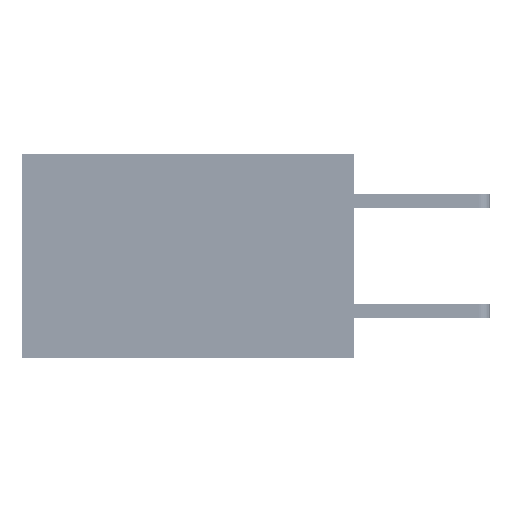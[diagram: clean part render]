
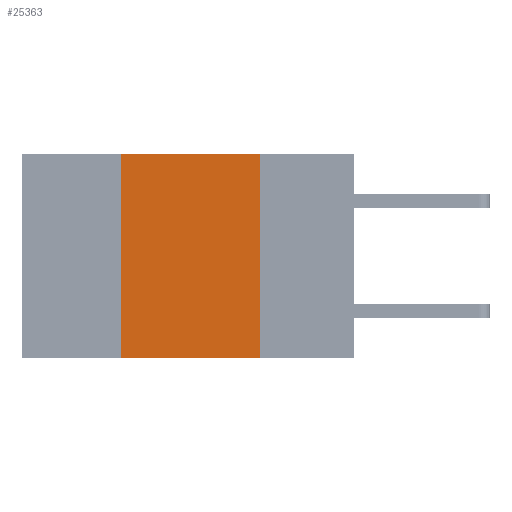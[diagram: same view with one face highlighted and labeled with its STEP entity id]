
A CAD part, left-side view. The second image highlights one B-rep face of the part: STEP entity #25363.
In plain terms, the highlighted planar face has unit normal (-1, 0, 0).
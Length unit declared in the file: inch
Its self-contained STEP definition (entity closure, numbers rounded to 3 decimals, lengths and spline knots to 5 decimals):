
#159 = EDGE_CURVE ( 'NONE', #47427, #36106, #2093, .T. ) ;
#1109 = VECTOR ( 'NONE', #7773, 39.37008 ) ;
#2093 = LINE ( 'NONE', #46073, #29118 ) ;
#7512 = VECTOR ( 'NONE', #10268, 39.37008 ) ;
#7773 = DIRECTION ( 'NONE',  ( 0., -1., 0. ) ) ;
#8421 = CARTESIAN_POINT ( 'NONE',  ( 0., 0.17, 0. ) ) ;
#10268 = DIRECTION ( 'NONE',  ( 0., 0., -1. ) ) ;
#12134 = VERTEX_POINT ( 'NONE', #36921 ) ;
#12725 = CARTESIAN_POINT ( 'NONE',  ( 0., 0.6, -0.37 ) ) ;
#14326 = DIRECTION ( 'NONE',  ( 1., 0., 0. ) ) ;
#14480 = EDGE_LOOP ( 'NONE', ( #38551, #17842, #36214, #17178 ) ) ;
#14865 = PLANE ( 'NONE',  #25245 ) ;
#14937 = LINE ( 'NONE', #27923, #1109 ) ;
#16442 = LINE ( 'NONE', #12725, #31491 ) ;
#17178 = ORIENTED_EDGE ( 'NONE', *, *, #31891, .T. ) ;
#17842 = ORIENTED_EDGE ( 'NONE', *, *, #32676, .F. ) ;
#25245 = AXIS2_PLACEMENT_3D ( 'NONE', #35526, #14326, #35260 ) ;
#25363 = ADVANCED_FACE ( 'NONE', ( #26541 ), #14865, .F. ) ;
#25878 = EDGE_CURVE ( 'NONE', #39779, #12134, #52161, .T. ) ;
#26541 = FACE_OUTER_BOUND ( 'NONE', #14480, .T. ) ;
#27923 = CARTESIAN_POINT ( 'NONE',  ( 0., 0.6, 0. ) ) ;
#29118 = VECTOR ( 'NONE', #42084, 39.37008 ) ;
#31491 = VECTOR ( 'NONE', #48502, 39.37008 ) ;
#31891 = EDGE_CURVE ( 'NONE', #47427, #12134, #16442, .T. ) ;
#32676 = EDGE_CURVE ( 'NONE', #36106, #39779, #14937, .T. ) ;
#34858 = CARTESIAN_POINT ( 'NONE',  ( 0., 0.17, 0. ) ) ;
#35260 = DIRECTION ( 'NONE',  ( 0., 0., -1. ) ) ;
#35526 = CARTESIAN_POINT ( 'NONE',  ( 0., 0.6, 0. ) ) ;
#36106 = VERTEX_POINT ( 'NONE', #51898 ) ;
#36214 = ORIENTED_EDGE ( 'NONE', *, *, #159, .F. ) ;
#36921 = CARTESIAN_POINT ( 'NONE',  ( 0., 0.17, -0.37 ) ) ;
#37912 = CARTESIAN_POINT ( 'NONE',  ( 0., 0.42, -0.37 ) ) ;
#38551 = ORIENTED_EDGE ( 'NONE', *, *, #25878, .F. ) ;
#39779 = VERTEX_POINT ( 'NONE', #34858 ) ;
#42084 = DIRECTION ( 'NONE',  ( 0., 0., 1. ) ) ;
#46073 = CARTESIAN_POINT ( 'NONE',  ( 0., 0.42, 0. ) ) ;
#47427 = VERTEX_POINT ( 'NONE', #37912 ) ;
#48502 = DIRECTION ( 'NONE',  ( 0., -1., 0. ) ) ;
#51898 = CARTESIAN_POINT ( 'NONE',  ( 0., 0.42, 0. ) ) ;
#52161 = LINE ( 'NONE', #8421, #7512 ) ;
